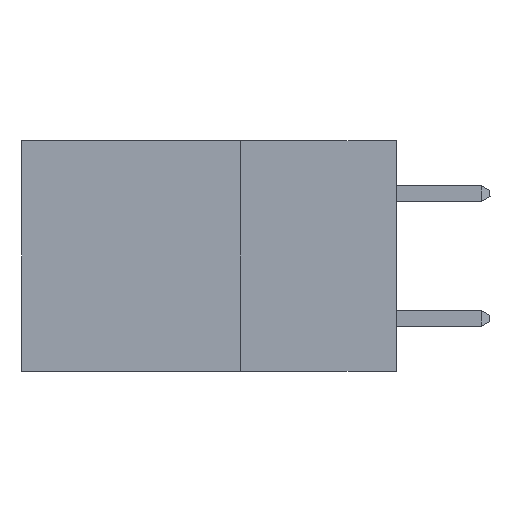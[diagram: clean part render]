
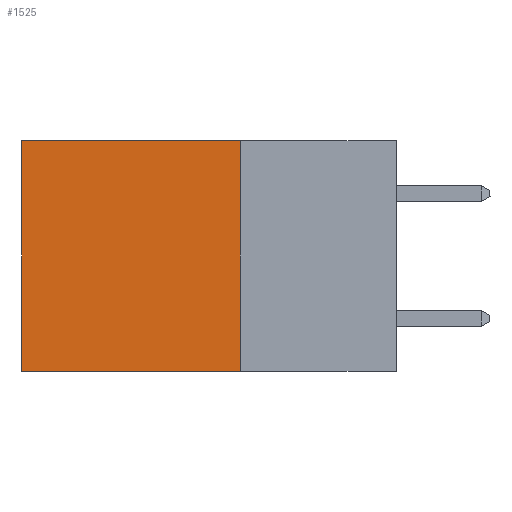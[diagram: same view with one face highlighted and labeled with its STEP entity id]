
A CAD part, left-side view. The second image highlights one B-rep face of the part: STEP entity #1525.
In plain terms, the highlighted planar face has unit normal (-1, 0, 0).
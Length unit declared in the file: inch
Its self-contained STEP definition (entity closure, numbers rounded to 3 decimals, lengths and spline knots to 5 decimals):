
#42 = ORIENTED_EDGE ( 'NONE', *, *, #8133, .T. ) ;
#88 = FACE_OUTER_BOUND ( 'NONE', #3444, .T. ) ;
#259 = ORIENTED_EDGE ( 'NONE', *, *, #15549, .F. ) ;
#733 = ORIENTED_EDGE ( 'NONE', *, *, #18920, .T. ) ;
#1525 = ADVANCED_FACE ( 'NONE', ( #88 ), #5928, .F. ) ;
#2537 = CARTESIAN_POINT ( 'NONE',  ( 0.298, 0.6, -0.37 ) ) ;
#2714 = AXIS2_PLACEMENT_3D ( 'NONE', #7411, #8825, #13048 ) ;
#2822 = LINE ( 'NONE', #4706, #18435 ) ;
#2893 = ORIENTED_EDGE ( 'NONE', *, *, #7491, .F. ) ;
#3444 = EDGE_LOOP ( 'NONE', ( #42, #2893, #259, #733 ) ) ;
#4706 = CARTESIAN_POINT ( 'NONE',  ( 0.298, 0.6, 0. ) ) ;
#5608 = CARTESIAN_POINT ( 'NONE',  ( 0.298, 0.25, 0. ) ) ;
#5928 = PLANE ( 'NONE',  #2714 ) ;
#6682 = VERTEX_POINT ( 'NONE', #7908 ) ;
#6916 = VECTOR ( 'NONE', #17335, 39.37008 ) ;
#7376 = LINE ( 'NONE', #5608, #6916 ) ;
#7411 = CARTESIAN_POINT ( 'NONE',  ( 0.298, 0.25, 0. ) ) ;
#7480 = VECTOR ( 'NONE', #14217, 39.37008 ) ;
#7491 = EDGE_CURVE ( 'NONE', #15878, #17178, #17698, .T. ) ;
#7908 = CARTESIAN_POINT ( 'NONE',  ( 0.298, 0.6, 0. ) ) ;
#8133 = EDGE_CURVE ( 'NONE', #6682, #17178, #2822, .T. ) ;
#8825 = DIRECTION ( 'NONE',  ( 1., 0., 0. ) ) ;
#10332 = VERTEX_POINT ( 'NONE', #16075 ) ;
#10432 = VECTOR ( 'NONE', #15263, 39.37008 ) ;
#12704 = CARTESIAN_POINT ( 'NONE',  ( 0.298, 0.25, -0.37 ) ) ;
#13048 = DIRECTION ( 'NONE',  ( 0., 0., -1. ) ) ;
#13928 = CARTESIAN_POINT ( 'NONE',  ( 0.298, 0.25, -0.37 ) ) ;
#14217 = DIRECTION ( 'NONE',  ( 0., 1., 0. ) ) ;
#15048 = DIRECTION ( 'NONE',  ( 0., 0., -1. ) ) ;
#15263 = DIRECTION ( 'NONE',  ( 0., 0., -1. ) ) ;
#15549 = EDGE_CURVE ( 'NONE', #10332, #15878, #17307, .T. ) ;
#15878 = VERTEX_POINT ( 'NONE', #13928 ) ;
#16075 = CARTESIAN_POINT ( 'NONE',  ( 0.298, 0.25, 0. ) ) ;
#17178 = VERTEX_POINT ( 'NONE', #2537 ) ;
#17307 = LINE ( 'NONE', #17973, #10432 ) ;
#17335 = DIRECTION ( 'NONE',  ( 0., 1., 0. ) ) ;
#17698 = LINE ( 'NONE', #12704, #7480 ) ;
#17973 = CARTESIAN_POINT ( 'NONE',  ( 0.298, 0.25, 0. ) ) ;
#18435 = VECTOR ( 'NONE', #15048, 39.37008 ) ;
#18920 = EDGE_CURVE ( 'NONE', #10332, #6682, #7376, .T. ) ;
